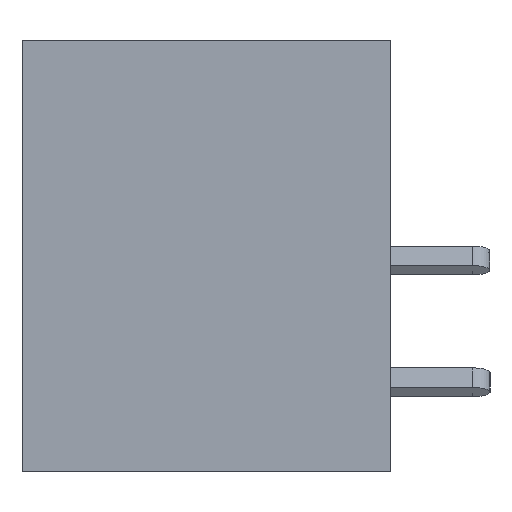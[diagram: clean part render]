
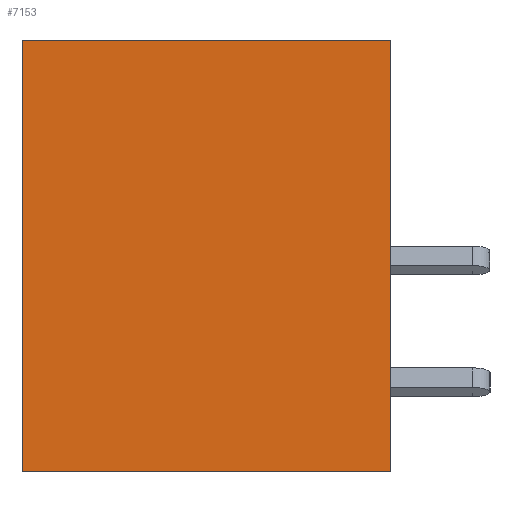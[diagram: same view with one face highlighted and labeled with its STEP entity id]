
A CAD part, left-side view. The second image highlights one B-rep face of the part: STEP entity #7153.
In plain terms, the highlighted planar face has unit normal (-1, 0, 0).
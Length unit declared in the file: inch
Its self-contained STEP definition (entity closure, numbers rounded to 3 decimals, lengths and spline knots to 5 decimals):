
#374 = VERTEX_POINT ( 'NONE', #19804 ) ;
#1490 = DIRECTION ( 'NONE',  ( 0., -1., 0. ) ) ;
#2330 = VECTOR ( 'NONE', #21001, 39.37008 ) ;
#3324 = LINE ( 'NONE', #12309, #2330 ) ;
#3658 = VERTEX_POINT ( 'NONE', #10138 ) ;
#4222 = VECTOR ( 'NONE', #10626, 39.37008 ) ;
#4284 = ORIENTED_EDGE ( 'NONE', *, *, #9023, .F. ) ;
#4928 = VERTEX_POINT ( 'NONE', #12935 ) ;
#5087 = PLANE ( 'NONE',  #15164 ) ;
#6231 = VECTOR ( 'NONE', #1490, 39.37008 ) ;
#6335 = CARTESIAN_POINT ( 'NONE',  ( 0., 0.453, -0.531 ) ) ;
#7153 = ADVANCED_FACE ( 'NONE', ( #25106 ), #5087, .F. ) ;
#9023 = EDGE_CURVE ( 'NONE', #24117, #3658, #14547, .T. ) ;
#9407 = CARTESIAN_POINT ( 'NONE',  ( 0., 0.453, 0. ) ) ;
#10138 = CARTESIAN_POINT ( 'NONE',  ( 0., 0.453, 0. ) ) ;
#10189 = CARTESIAN_POINT ( 'NONE',  ( 0., 0.453, 0. ) ) ;
#10626 = DIRECTION ( 'NONE',  ( 0., -1., 0. ) ) ;
#10771 = EDGE_CURVE ( 'NONE', #3658, #374, #11908, .T. ) ;
#11908 = LINE ( 'NONE', #21211, #6231 ) ;
#12309 = CARTESIAN_POINT ( 'NONE',  ( 0., 0., 0. ) ) ;
#12738 = ORIENTED_EDGE ( 'NONE', *, *, #10771, .F. ) ;
#12859 = VECTOR ( 'NONE', #22993, 39.37008 ) ;
#12935 = CARTESIAN_POINT ( 'NONE',  ( 0., 0., -0.531 ) ) ;
#14547 = LINE ( 'NONE', #10189, #12859 ) ;
#14836 = EDGE_CURVE ( 'NONE', #4928, #374, #3324, .T. ) ;
#15164 = AXIS2_PLACEMENT_3D ( 'NONE', #9407, #16180, #18061 ) ;
#16180 = DIRECTION ( 'NONE',  ( 1., 0., 0. ) ) ;
#18061 = DIRECTION ( 'NONE',  ( 0., 0., -1. ) ) ;
#18816 = EDGE_CURVE ( 'NONE', #24117, #4928, #23400, .T. ) ;
#19175 = ORIENTED_EDGE ( 'NONE', *, *, #14836, .T. ) ;
#19804 = CARTESIAN_POINT ( 'NONE',  ( 0., 0., 0. ) ) ;
#21001 = DIRECTION ( 'NONE',  ( 0., 0., 1. ) ) ;
#21211 = CARTESIAN_POINT ( 'NONE',  ( 0., 0.453, 0. ) ) ;
#22993 = DIRECTION ( 'NONE',  ( 0., 0., 1. ) ) ;
#23400 = LINE ( 'NONE', #6335, #4222 ) ;
#24117 = VERTEX_POINT ( 'NONE', #27829 ) ;
#24908 = EDGE_LOOP ( 'NONE', ( #19175, #12738, #4284, #26219 ) ) ;
#25106 = FACE_OUTER_BOUND ( 'NONE', #24908, .T. ) ;
#26219 = ORIENTED_EDGE ( 'NONE', *, *, #18816, .T. ) ;
#27829 = CARTESIAN_POINT ( 'NONE',  ( 0., 0.453, -0.531 ) ) ;
